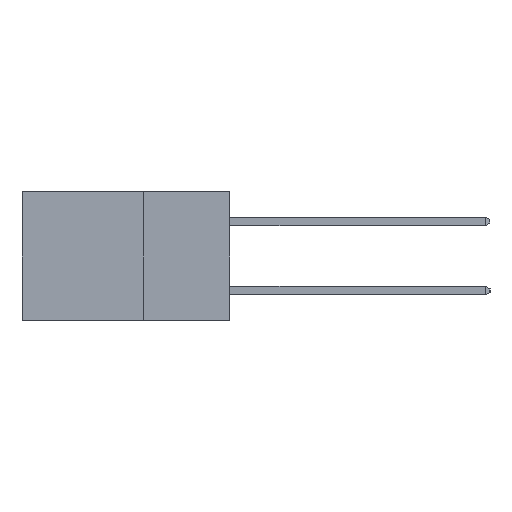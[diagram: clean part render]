
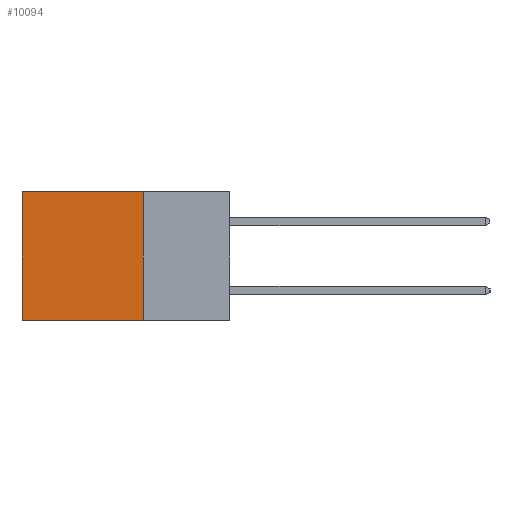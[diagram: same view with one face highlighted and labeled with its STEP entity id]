
A CAD part, left-side view. The second image highlights one B-rep face of the part: STEP entity #10094.
In plain terms, the highlighted planar face has unit normal (-1, 0, 0).
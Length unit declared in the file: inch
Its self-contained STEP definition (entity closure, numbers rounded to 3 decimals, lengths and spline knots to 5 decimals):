
#40 = ORIENTED_EDGE ( 'NONE', *, *, #890, .F. ) ;
#93 = VECTOR ( 'NONE', #1884, 39.37008 ) ;
#152 = VERTEX_POINT ( 'NONE', #9796 ) ;
#300 = AXIS2_PLACEMENT_3D ( 'NONE', #7368, #10999, #5545 ) ;
#545 = ORIENTED_EDGE ( 'NONE', *, *, #6384, .T. ) ;
#860 = CARTESIAN_POINT ( 'NONE',  ( 0.2615, 0.25, 0. ) ) ;
#890 = EDGE_CURVE ( 'NONE', #152, #5350, #6821, .T. ) ;
#1391 = CARTESIAN_POINT ( 'NONE',  ( 0.2615, 0.25, -0.37 ) ) ;
#1884 = DIRECTION ( 'NONE',  ( 0., 1., 0. ) ) ;
#2392 = DIRECTION ( 'NONE',  ( 0., 0., -1. ) ) ;
#2740 = LINE ( 'NONE', #860, #93 ) ;
#3154 = EDGE_LOOP ( 'NONE', ( #545, #40, #10197, #3536 ) ) ;
#3247 = FACE_OUTER_BOUND ( 'NONE', #3154, .T. ) ;
#3519 = VERTEX_POINT ( 'NONE', #8768 ) ;
#3536 = ORIENTED_EDGE ( 'NONE', *, *, #6734, .T. ) ;
#4595 = PLANE ( 'NONE',  #300 ) ;
#4779 = LINE ( 'NONE', #1391, #11759 ) ;
#4973 = VERTEX_POINT ( 'NONE', #11564 ) ;
#5274 = DIRECTION ( 'NONE',  ( 0., 1., 0. ) ) ;
#5350 = VERTEX_POINT ( 'NONE', #6871 ) ;
#5545 = DIRECTION ( 'NONE',  ( 0., 0., -1. ) ) ;
#6053 = CARTESIAN_POINT ( 'NONE',  ( 0.2615, 0.25, -0.37 ) ) ;
#6384 = EDGE_CURVE ( 'NONE', #4973, #5350, #9324, .T. ) ;
#6734 = EDGE_CURVE ( 'NONE', #3519, #4973, #2740, .T. ) ;
#6821 = LINE ( 'NONE', #6053, #11343 ) ;
#6871 = CARTESIAN_POINT ( 'NONE',  ( 0.2615, 0.6, -0.37 ) ) ;
#6907 = VECTOR ( 'NONE', #2392, 39.37008 ) ;
#7151 = DIRECTION ( 'NONE',  ( 0., 0., -1. ) ) ;
#7368 = CARTESIAN_POINT ( 'NONE',  ( 0.2615, 0.25, -0.37 ) ) ;
#8054 = CARTESIAN_POINT ( 'NONE',  ( 0.2615, 0.6, -0.37 ) ) ;
#8768 = CARTESIAN_POINT ( 'NONE',  ( 0.2615, 0.25, 0. ) ) ;
#9196 = EDGE_CURVE ( 'NONE', #3519, #152, #4779, .T. ) ;
#9324 = LINE ( 'NONE', #8054, #6907 ) ;
#9796 = CARTESIAN_POINT ( 'NONE',  ( 0.2615, 0.25, -0.37 ) ) ;
#10094 = ADVANCED_FACE ( 'NONE', ( #3247 ), #4595, .F. ) ;
#10197 = ORIENTED_EDGE ( 'NONE', *, *, #9196, .F. ) ;
#10999 = DIRECTION ( 'NONE',  ( 1., 0., 0. ) ) ;
#11343 = VECTOR ( 'NONE', #5274, 39.37008 ) ;
#11564 = CARTESIAN_POINT ( 'NONE',  ( 0.2615, 0.6, 0. ) ) ;
#11759 = VECTOR ( 'NONE', #7151, 39.37008 ) ;
